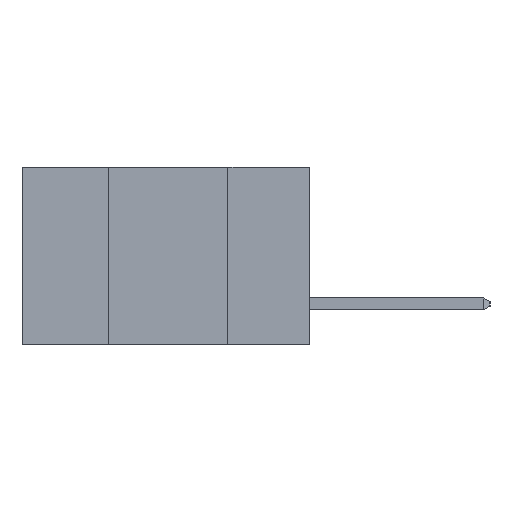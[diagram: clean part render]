
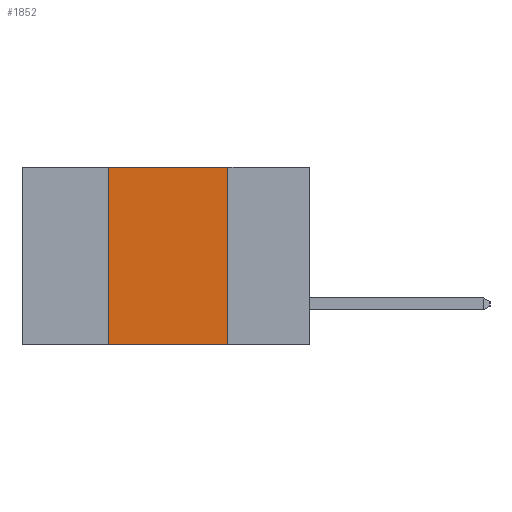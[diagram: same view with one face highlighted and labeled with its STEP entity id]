
A CAD part, left-side view. The second image highlights one B-rep face of the part: STEP entity #1852.
In plain terms, the highlighted planar face has unit normal (-1, 0, 0).
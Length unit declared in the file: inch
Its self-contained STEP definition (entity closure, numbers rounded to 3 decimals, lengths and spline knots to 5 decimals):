
#1351 = VECTOR ( 'NONE', #9584, 39.37008 ) ;
#1852 = ADVANCED_FACE ( 'NONE', ( #11174 ), #17533, .F. ) ;
#1907 = ORIENTED_EDGE ( 'NONE', *, *, #13841, .F. ) ;
#3347 = DIRECTION ( 'NONE',  ( 0., 0., -1. ) ) ;
#3801 = DIRECTION ( 'NONE',  ( 0., -1., 0. ) ) ;
#3983 = LINE ( 'NONE', #19547, #14225 ) ;
#4080 = VERTEX_POINT ( 'NONE', #20331 ) ;
#4300 = LINE ( 'NONE', #10840, #1351 ) ;
#4816 = CARTESIAN_POINT ( 'NONE',  ( 0., 0.6, 0. ) ) ;
#4864 = ORIENTED_EDGE ( 'NONE', *, *, #15995, .F. ) ;
#5006 = EDGE_CURVE ( 'NONE', #19292, #4080, #4300, .T. ) ;
#5090 = LINE ( 'NONE', #14867, #6089 ) ;
#6089 = VECTOR ( 'NONE', #17934, 39.37008 ) ;
#6645 = EDGE_LOOP ( 'NONE', ( #20526, #4864, #1907, #20183 ) ) ;
#6856 = CARTESIAN_POINT ( 'NONE',  ( 0., 0.42, 0. ) ) ;
#8627 = VERTEX_POINT ( 'NONE', #6856 ) ;
#9584 = DIRECTION ( 'NONE',  ( 0., -1., 0. ) ) ;
#10484 = EDGE_CURVE ( 'NONE', #11390, #4080, #14193, .T. ) ;
#10840 = CARTESIAN_POINT ( 'NONE',  ( 0., 0.6, -0.37 ) ) ;
#11174 = FACE_OUTER_BOUND ( 'NONE', #6645, .T. ) ;
#11390 = VERTEX_POINT ( 'NONE', #19577 ) ;
#12607 = DIRECTION ( 'NONE',  ( 0., 0., -1. ) ) ;
#12908 = VECTOR ( 'NONE', #12607, 39.37008 ) ;
#13841 = EDGE_CURVE ( 'NONE', #19292, #8627, #5090, .T. ) ;
#14193 = LINE ( 'NONE', #18943, #12908 ) ;
#14225 = VECTOR ( 'NONE', #3801, 39.37008 ) ;
#14553 = CARTESIAN_POINT ( 'NONE',  ( 0., 0.42, -0.37 ) ) ;
#14867 = CARTESIAN_POINT ( 'NONE',  ( 0., 0.42, 0. ) ) ;
#15995 = EDGE_CURVE ( 'NONE', #8627, #11390, #3983, .T. ) ;
#16859 = AXIS2_PLACEMENT_3D ( 'NONE', #4816, #19572, #3347 ) ;
#17533 = PLANE ( 'NONE',  #16859 ) ;
#17934 = DIRECTION ( 'NONE',  ( 0., 0., 1. ) ) ;
#18943 = CARTESIAN_POINT ( 'NONE',  ( 0., 0.17, 0. ) ) ;
#19292 = VERTEX_POINT ( 'NONE', #14553 ) ;
#19547 = CARTESIAN_POINT ( 'NONE',  ( 0., 0.6, 0. ) ) ;
#19572 = DIRECTION ( 'NONE',  ( 1., 0., 0. ) ) ;
#19577 = CARTESIAN_POINT ( 'NONE',  ( 0., 0.17, 0. ) ) ;
#20183 = ORIENTED_EDGE ( 'NONE', *, *, #5006, .T. ) ;
#20331 = CARTESIAN_POINT ( 'NONE',  ( 0., 0.17, -0.37 ) ) ;
#20526 = ORIENTED_EDGE ( 'NONE', *, *, #10484, .F. ) ;
